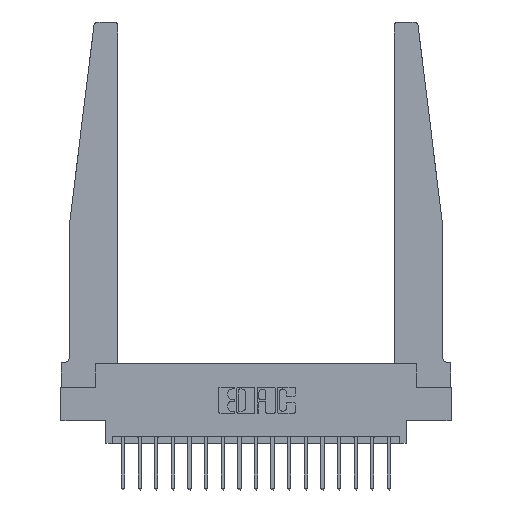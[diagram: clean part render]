
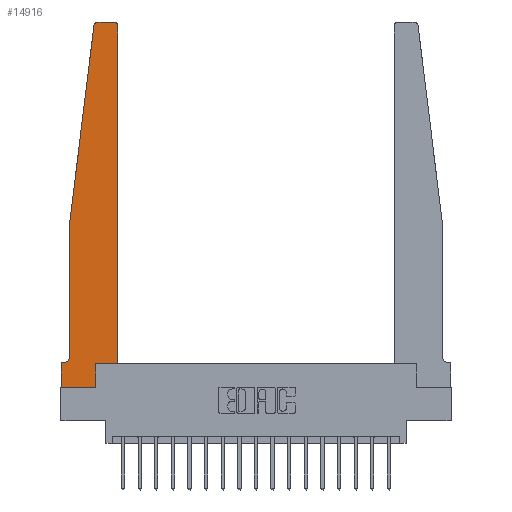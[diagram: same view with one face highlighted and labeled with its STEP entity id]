
A CAD part, top view. The second image highlights one B-rep face of the part: STEP entity #14916.
In plain terms, the highlighted planar face has unit normal (0, 0, 1).
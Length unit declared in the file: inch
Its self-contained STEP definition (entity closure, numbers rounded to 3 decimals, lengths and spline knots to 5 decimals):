
#235 = CARTESIAN_POINT ( 'NONE',  ( 0., 0.1875, 0.37 ) ) ;
#515 = VECTOR ( 'NONE', #2074, 39.37008 ) ;
#760 = VERTEX_POINT ( 'NONE', #13535 ) ;
#825 = DIRECTION ( 'NONE',  ( 1., 0., 0. ) ) ;
#1025 = CARTESIAN_POINT ( 'NONE',  ( 0.24675, 2.72367, 0.37 ) ) ;
#1527 = CARTESIAN_POINT ( 'NONE',  ( 0.425, 0.18, 0.37 ) ) ;
#1745 = CARTESIAN_POINT ( 'NONE',  ( 0.2605, 0., 0.37 ) ) ;
#1975 = VERTEX_POINT ( 'NONE', #2317 ) ;
#2074 = DIRECTION ( 'NONE',  ( 0., 1., 0. ) ) ;
#2253 = DIRECTION ( 'NONE',  ( 0., 0., -1. ) ) ;
#2317 = CARTESIAN_POINT ( 'NONE',  ( 0.425, 0.18, 0.37 ) ) ;
#2320 = VERTEX_POINT ( 'NONE', #13810 ) ;
#2360 = EDGE_LOOP ( 'NONE', ( #11446, #11710, #11751, #12275, #12595, #13725, #14568, #16433, #17275, #17405, #17513, #17881 ) ) ;
#3125 = VERTEX_POINT ( 'NONE', #12799 ) ;
#3302 = AXIS2_PLACEMENT_3D ( 'NONE', #5475, #15964, #7000 ) ;
#3513 = VERTEX_POINT ( 'NONE', #1745 ) ;
#3652 = LINE ( 'NONE', #9822, #15620 ) ;
#3892 = AXIS2_PLACEMENT_3D ( 'NONE', #16173, #7219, #17662 ) ;
#4176 = PLANE ( 'NONE',  #15198 ) ;
#5023 = EDGE_CURVE ( 'NONE', #3125, #6366, #13965, .T. ) ;
#5204 = CARTESIAN_POINT ( 'NONE',  ( 0.065, 1.25, 0.37 ) ) ;
#5307 = VERTEX_POINT ( 'NONE', #235 ) ;
#5475 = CARTESIAN_POINT ( 'NONE',  ( 0.27653, 2.72, 0.37 ) ) ;
#5495 = LINE ( 'NONE', #15492, #12538 ) ;
#5850 = VECTOR ( 'NONE', #6068, 39.37008 ) ;
#6068 = DIRECTION ( 'NONE',  ( 0., 1., 0. ) ) ;
#6334 = LINE ( 'NONE', #1527, #5850 ) ;
#6366 = VERTEX_POINT ( 'NONE', #7591 ) ;
#6370 = CARTESIAN_POINT ( 'NONE',  ( 0.25, 2.75, 0.37 ) ) ;
#6600 = EDGE_CURVE ( 'NONE', #3513, #2320, #12485, .T. ) ;
#6628 = CARTESIAN_POINT ( 'NONE',  ( 0.425, 0.18, 0.37 ) ) ;
#7000 = DIRECTION ( 'NONE',  ( 1., 0., 0. ) ) ;
#7219 = DIRECTION ( 'NONE',  ( 0., 0., 1. ) ) ;
#7233 = DIRECTION ( 'NONE',  ( 1., 0., 0. ) ) ;
#7380 = EDGE_CURVE ( 'NONE', #19264, #12082, #7809, .T. ) ;
#7465 = EDGE_CURVE ( 'NONE', #760, #11629, #14796, .T. ) ;
#7591 = CARTESIAN_POINT ( 'NONE',  ( 0.395, 2.75, 0.37 ) ) ;
#7809 = CIRCLE ( 'NONE', #17728, 0.05 ) ;
#7903 = DIRECTION ( 'NONE',  ( -1., 0., 0. ) ) ;
#8180 = DIRECTION ( 'NONE',  ( 0., -1., 0. ) ) ;
#8309 = EDGE_CURVE ( 'NONE', #11629, #17297, #9174, .T. ) ;
#8538 = EDGE_CURVE ( 'NONE', #1975, #3125, #6334, .T. ) ;
#9174 = LINE ( 'NONE', #5204, #17080 ) ;
#9224 = CARTESIAN_POINT ( 'NONE',  ( 0.065, 0.2375, 0.37 ) ) ;
#9333 = EDGE_CURVE ( 'NONE', #6366, #760, #16588, .T. ) ;
#9822 = CARTESIAN_POINT ( 'NONE',  ( 0., 0., 0.37 ) ) ;
#10323 = VERTEX_POINT ( 'NONE', #11908 ) ;
#11110 = DIRECTION ( 'NONE',  ( -1., 0., 0. ) ) ;
#11272 = CARTESIAN_POINT ( 'NONE',  ( 0.015, 0.2375, 0.37 ) ) ;
#11446 = ORIENTED_EDGE ( 'NONE', *, *, #9333, .T. ) ;
#11629 = VERTEX_POINT ( 'NONE', #1025 ) ;
#11710 = ORIENTED_EDGE ( 'NONE', *, *, #7465, .T. ) ;
#11751 = ORIENTED_EDGE ( 'NONE', *, *, #8309, .T. ) ;
#11908 = CARTESIAN_POINT ( 'NONE',  ( 0., 0., 0.37 ) ) ;
#11940 = EDGE_CURVE ( 'NONE', #10323, #3513, #3652, .T. ) ;
#12011 = VECTOR ( 'NONE', #14088, 39.37008 ) ;
#12082 = VERTEX_POINT ( 'NONE', #14587 ) ;
#12275 = ORIENTED_EDGE ( 'NONE', *, *, #18101, .T. ) ;
#12407 = EDGE_CURVE ( 'NONE', #12082, #5307, #15602, .T. ) ;
#12485 = LINE ( 'NONE', #17020, #515 ) ;
#12538 = VECTOR ( 'NONE', #15557, 39.37008 ) ;
#12595 = ORIENTED_EDGE ( 'NONE', *, *, #7380, .T. ) ;
#12713 = FACE_OUTER_BOUND ( 'NONE', #2360, .T. ) ;
#12770 = DIRECTION ( 'NONE',  ( -1., 0., 0. ) ) ;
#12799 = CARTESIAN_POINT ( 'NONE',  ( 0.425, 2.72, 0.37 ) ) ;
#13535 = CARTESIAN_POINT ( 'NONE',  ( 0.27653, 2.75, 0.37 ) ) ;
#13725 = ORIENTED_EDGE ( 'NONE', *, *, #12407, .T. ) ;
#13810 = CARTESIAN_POINT ( 'NONE',  ( 0.2605, 0.18, 0.37 ) ) ;
#13965 = CIRCLE ( 'NONE', #3892, 0.03 ) ;
#14088 = DIRECTION ( 'NONE',  ( 1., 0., 0. ) ) ;
#14568 = ORIENTED_EDGE ( 'NONE', *, *, #17028, .T. ) ;
#14587 = CARTESIAN_POINT ( 'NONE',  ( 0.015, 0.1875, 0.37 ) ) ;
#14796 = CIRCLE ( 'NONE', #3302, 0.03 ) ;
#14916 = ADVANCED_FACE ( 'NONE', ( #12713 ), #4176, .T. ) ;
#15147 = VECTOR ( 'NONE', #11110, 39.37008 ) ;
#15187 = EDGE_CURVE ( 'NONE', #2320, #1975, #16892, .T. ) ;
#15198 = AXIS2_PLACEMENT_3D ( 'NONE', #17611, #16184, #7233 ) ;
#15492 = CARTESIAN_POINT ( 'NONE',  ( 0.065, 1.25, 0.37 ) ) ;
#15539 = CARTESIAN_POINT ( 'NONE',  ( 0.065, 0.1875, 0.37 ) ) ;
#15557 = DIRECTION ( 'NONE',  ( 0., -1., 0. ) ) ;
#15597 = CARTESIAN_POINT ( 'NONE',  ( 0., 0., 0.37 ) ) ;
#15602 = LINE ( 'NONE', #15539, #15147 ) ;
#15620 = VECTOR ( 'NONE', #825, 39.37008 ) ;
#15686 = DIRECTION ( 'NONE',  ( -0.122, -0.992, 0. ) ) ;
#15964 = DIRECTION ( 'NONE',  ( 0., 0., 1. ) ) ;
#16128 = VECTOR ( 'NONE', #7903, 39.37008 ) ;
#16173 = CARTESIAN_POINT ( 'NONE',  ( 0.395, 2.72, 0.37 ) ) ;
#16184 = DIRECTION ( 'NONE',  ( 0., 0., 1. ) ) ;
#16363 = LINE ( 'NONE', #15597, #16822 ) ;
#16433 = ORIENTED_EDGE ( 'NONE', *, *, #11940, .T. ) ;
#16588 = LINE ( 'NONE', #6370, #16128 ) ;
#16822 = VECTOR ( 'NONE', #8180, 39.37008 ) ;
#16892 = LINE ( 'NONE', #6628, #12011 ) ;
#17020 = CARTESIAN_POINT ( 'NONE',  ( 0.2605, 0.18, 0.37 ) ) ;
#17028 = EDGE_CURVE ( 'NONE', #5307, #10323, #16363, .T. ) ;
#17080 = VECTOR ( 'NONE', #15686, 39.37008 ) ;
#17275 = ORIENTED_EDGE ( 'NONE', *, *, #6600, .T. ) ;
#17297 = VERTEX_POINT ( 'NONE', #19357 ) ;
#17405 = ORIENTED_EDGE ( 'NONE', *, *, #15187, .T. ) ;
#17513 = ORIENTED_EDGE ( 'NONE', *, *, #8538, .T. ) ;
#17611 = CARTESIAN_POINT ( 'NONE',  ( 0., 0.1875, 0.37 ) ) ;
#17662 = DIRECTION ( 'NONE',  ( 1., 0., 0. ) ) ;
#17728 = AXIS2_PLACEMENT_3D ( 'NONE', #11272, #2253, #12770 ) ;
#17881 = ORIENTED_EDGE ( 'NONE', *, *, #5023, .T. ) ;
#18101 = EDGE_CURVE ( 'NONE', #17297, #19264, #5495, .T. ) ;
#19264 = VERTEX_POINT ( 'NONE', #9224 ) ;
#19357 = CARTESIAN_POINT ( 'NONE',  ( 0.065, 1.25, 0.37 ) ) ;
